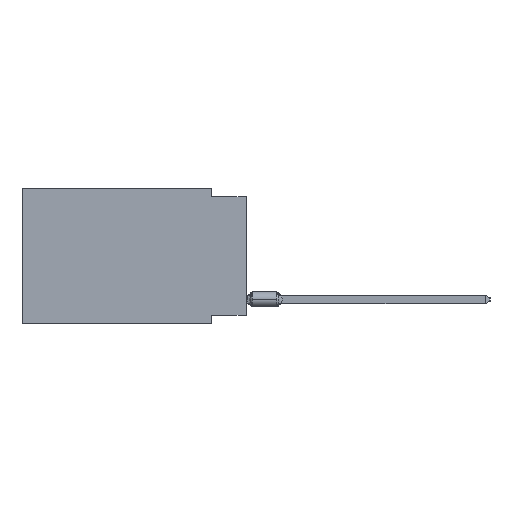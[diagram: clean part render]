
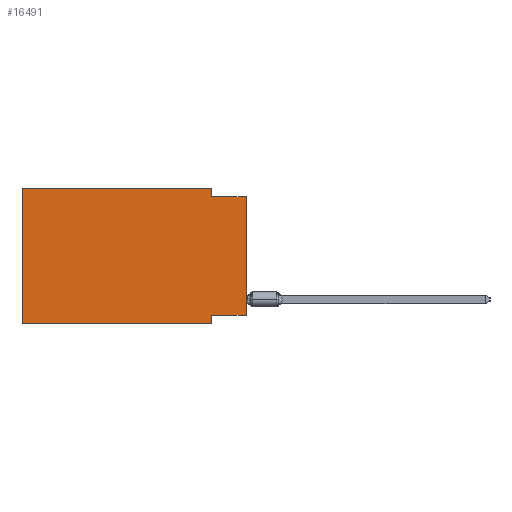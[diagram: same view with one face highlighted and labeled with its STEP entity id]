
A CAD part, left-side view. The second image highlights one B-rep face of the part: STEP entity #16491.
In plain terms, the highlighted planar face has unit normal (-1, 0, 0).
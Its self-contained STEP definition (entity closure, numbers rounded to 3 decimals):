
#958 = ORIENTED_EDGE ( 'NONE', *, *, #9856, .F. ) ;
#1152 = EDGE_CURVE ( 'NONE', #13160, #22457, #27671, .T. ) ;
#1763 = DIRECTION ( 'NONE',  ( 0., 0., 1. ) ) ;
#1865 = ORIENTED_EDGE ( 'NONE', *, *, #7199, .F. ) ;
#2426 = CARTESIAN_POINT ( 'NONE',  ( 0., 2.54, 0. ) ) ;
#3477 = LINE ( 'NONE', #18652, #21194 ) ;
#3738 = ORIENTED_EDGE ( 'NONE', *, *, #32026, .F. ) ;
#4148 = EDGE_CURVE ( 'NONE', #43800, #35298, #23459, .T. ) ;
#4372 = EDGE_CURVE ( 'NONE', #37620, #36580, #35950, .T. ) ;
#6096 = DIRECTION ( 'NONE',  ( 0., -1., 0. ) ) ;
#7199 = EDGE_CURVE ( 'NONE', #35298, #37620, #21744, .T. ) ;
#7551 = EDGE_CURVE ( 'NONE', #43800, #45363, #41015, .T. ) ;
#8793 = VERTEX_POINT ( 'NONE', #20860 ) ;
#9856 = EDGE_CURVE ( 'NONE', #13160, #8793, #26320, .T. ) ;
#10334 = CARTESIAN_POINT ( 'NONE',  ( 0., 2.54, -9.906 ) ) ;
#11399 = DIRECTION ( 'NONE',  ( 0., 1., 0. ) ) ;
#11451 = CARTESIAN_POINT ( 'NONE',  ( 0., 2.54, 0. ) ) ;
#11854 = CARTESIAN_POINT ( 'NONE',  ( 0., 16.383, -9.906 ) ) ;
#12257 = VECTOR ( 'NONE', #43548, 1000. ) ;
#12399 = VECTOR ( 'NONE', #6096, 1000. ) ;
#13160 = VERTEX_POINT ( 'NONE', #19953 ) ;
#14306 = CARTESIAN_POINT ( 'NONE',  ( 0., 16.383, -9.906 ) ) ;
#15787 = CARTESIAN_POINT ( 'NONE',  ( 0., 16.383, 0. ) ) ;
#15898 = CARTESIAN_POINT ( 'NONE',  ( 0., 16.383, 0. ) ) ;
#15938 = CARTESIAN_POINT ( 'NONE',  ( 0., 0., 0. ) ) ;
#16491 = ADVANCED_FACE ( 'NONE', ( #30039 ), #30274, .F. ) ;
#17432 = AXIS2_PLACEMENT_3D ( 'NONE', #44991, #38119, #26827 ) ;
#18401 = DIRECTION ( 'NONE',  ( 0., 0., -1. ) ) ;
#18652 = CARTESIAN_POINT ( 'NONE',  ( 0., 2.54, -9.906 ) ) ;
#19081 = ORIENTED_EDGE ( 'NONE', *, *, #30887, .F. ) ;
#19953 = CARTESIAN_POINT ( 'NONE',  ( 0., 0., -9.271 ) ) ;
#20860 = CARTESIAN_POINT ( 'NONE',  ( 0., 2.54, -9.271 ) ) ;
#20998 = VECTOR ( 'NONE', #23091, 1000. ) ;
#21111 = ORIENTED_EDGE ( 'NONE', *, *, #4148, .F. ) ;
#21122 = VECTOR ( 'NONE', #37021, 1000. ) ;
#21194 = VECTOR ( 'NONE', #18401, 1000. ) ;
#21744 = LINE ( 'NONE', #36687, #12399 ) ;
#22317 = CARTESIAN_POINT ( 'NONE',  ( 0., 0., -0.635 ) ) ;
#22457 = VERTEX_POINT ( 'NONE', #25504 ) ;
#22753 = VECTOR ( 'NONE', #11399, 1000. ) ;
#23091 = DIRECTION ( 'NONE',  ( 0., -1., 0. ) ) ;
#23239 = ORIENTED_EDGE ( 'NONE', *, *, #4372, .F. ) ;
#23459 = LINE ( 'NONE', #15898, #44318 ) ;
#25504 = CARTESIAN_POINT ( 'NONE',  ( 0., 0., -0.635 ) ) ;
#26320 = LINE ( 'NONE', #26808, #22753 ) ;
#26808 = CARTESIAN_POINT ( 'NONE',  ( 0., 0., -9.271 ) ) ;
#26827 = DIRECTION ( 'NONE',  ( 0., 0., -1. ) ) ;
#27215 = ORIENTED_EDGE ( 'NONE', *, *, #1152, .T. ) ;
#27671 = LINE ( 'NONE', #15938, #30019 ) ;
#30019 = VECTOR ( 'NONE', #1763, 1000. ) ;
#30039 = FACE_OUTER_BOUND ( 'NONE', #44620, .T. ) ;
#30274 = PLANE ( 'NONE',  #17432 ) ;
#30887 = EDGE_CURVE ( 'NONE', #8793, #45363, #3477, .T. ) ;
#32026 = EDGE_CURVE ( 'NONE', #36580, #22457, #41184, .T. ) ;
#33775 = DIRECTION ( 'NONE',  ( 0., 0., 1. ) ) ;
#35298 = VERTEX_POINT ( 'NONE', #15787 ) ;
#35950 = LINE ( 'NONE', #2426, #12257 ) ;
#36580 = VERTEX_POINT ( 'NONE', #38814 ) ;
#36687 = CARTESIAN_POINT ( 'NONE',  ( 0., 16.383, 0. ) ) ;
#37021 = DIRECTION ( 'NONE',  ( 0., -1., 0. ) ) ;
#37620 = VERTEX_POINT ( 'NONE', #11451 ) ;
#38119 = DIRECTION ( 'NONE',  ( 1., 0., 0. ) ) ;
#38814 = CARTESIAN_POINT ( 'NONE',  ( 0., 2.54, -0.635 ) ) ;
#41015 = LINE ( 'NONE', #11854, #20998 ) ;
#41184 = LINE ( 'NONE', #22317, #21122 ) ;
#43548 = DIRECTION ( 'NONE',  ( 0., 0., -1. ) ) ;
#43800 = VERTEX_POINT ( 'NONE', #14306 ) ;
#44318 = VECTOR ( 'NONE', #33775, 1000. ) ;
#44395 = ORIENTED_EDGE ( 'NONE', *, *, #7551, .T. ) ;
#44620 = EDGE_LOOP ( 'NONE', ( #27215, #3738, #23239, #1865, #21111, #44395, #19081, #958 ) ) ;
#44991 = CARTESIAN_POINT ( 'NONE',  ( 0., 16.383, 0. ) ) ;
#45363 = VERTEX_POINT ( 'NONE', #10334 ) ;
